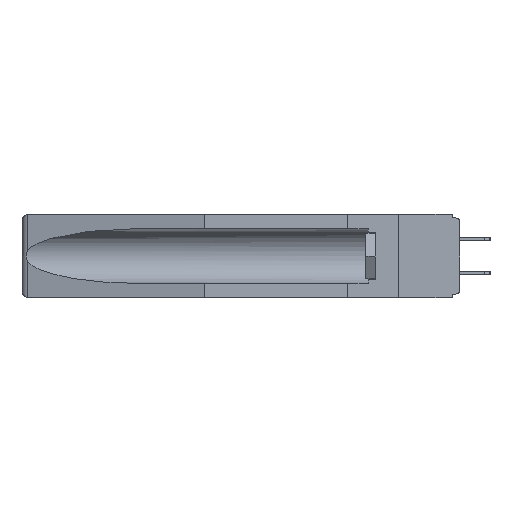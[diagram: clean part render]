
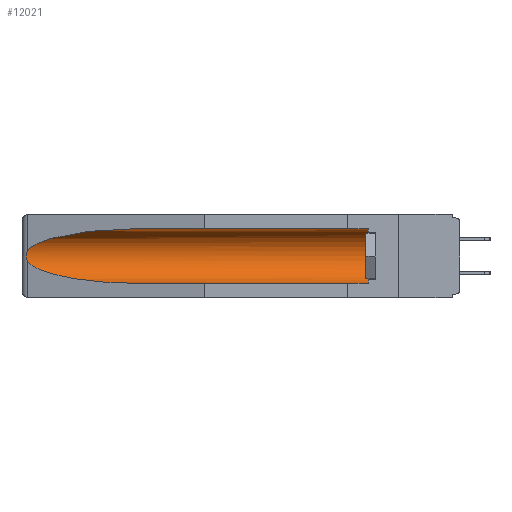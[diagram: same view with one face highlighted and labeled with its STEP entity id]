
A CAD part, left-side view. The second image highlights one B-rep face of the part: STEP entity #12021.
In plain terms, the highlighted cylindrical face has radius 2.857 mm (diameter 5.715 mm), a partial arc.
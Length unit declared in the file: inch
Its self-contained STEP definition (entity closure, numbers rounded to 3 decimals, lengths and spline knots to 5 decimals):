
#26 = EDGE_CURVE ( 'NONE', #24236, #4493, #21362, .T. ) ;
#445 = CARTESIAN_POINT ( 'NONE',  ( 0.155, 1.07973, -0.284 ) ) ;
#746 = DIRECTION ( 'NONE',  ( 0., -1., 0. ) ) ;
#1414 = AXIS2_PLACEMENT_3D ( 'NONE', #9236, #23745, #15819 ) ;
#2768 = CARTESIAN_POINT ( 'NONE',  ( 0.26597, 1.52961, -0.15275 ) ) ;
#2836 = CARTESIAN_POINT ( 'NONE',  ( 0.155, 1.07973, -0.059 ) ) ;
#3999 = DIRECTION ( 'NONE',  ( 0., 1., 0. ) ) ;
#4385 = CARTESIAN_POINT ( 'NONE',  ( 0.21114, 1.30732, -0.284 ) ) ;
#4493 = VERTEX_POINT ( 'NONE', #20191 ) ;
#4826 = CARTESIAN_POINT ( 'NONE',  ( 0.26537, 1.52718, -0.19328 ) ) ;
#4852 = CARTESIAN_POINT ( 'NONE',  ( 0.26537, 1.52718, -0.14972 ) ) ;
#5412 =( BOUNDED_CURVE ( )  B_SPLINE_CURVE ( 3, ( #15020, #23049, #4385, #445 ),
 .UNSPECIFIED., .F., .F. ) 
 B_SPLINE_CURVE_WITH_KNOTS ( ( 4, 4 ),
 ( 0.1948, 1.5708 ),
 .UNSPECIFIED. ) 
 CURVE ( )  GEOMETRIC_REPRESENTATION_ITEM ( )  RATIONAL_B_SPLINE_CURVE ( ( 1., 0.848, 0.848, 1. ) ) 
 REPRESENTATION_ITEM ( '' )  );
#5918 = CARTESIAN_POINT ( 'NONE',  ( 0.26537, 1.52718, -0.14972 ) ) ;
#6264 = ORIENTED_EDGE ( 'NONE', *, *, #21373, .T. ) ;
#7040 = VERTEX_POINT ( 'NONE', #2836 ) ;
#7216 = CARTESIAN_POINT ( 'NONE',  ( 0.155, 0.126, -0.284 ) ) ;
#7386 = ORIENTED_EDGE ( 'NONE', *, *, #23811, .F. ) ;
#8294 = VECTOR ( 'NONE', #3999, 39.37008 ) ;
#8612 = CARTESIAN_POINT ( 'NONE',  ( 0.26597, 1.5296, -0.19026 ) ) ;
#9236 = CARTESIAN_POINT ( 'NONE',  ( 0.155, -0.30754, -0.1715 ) ) ;
#9260 = CARTESIAN_POINT ( 'NONE',  ( 0.25451, 1.48313, -0.09465 ) ) ;
#9702 = ORIENTED_EDGE ( 'NONE', *, *, #26132, .T. ) ;
#9833 = CARTESIAN_POINT ( 'NONE',  ( 0.155, -0.30754, -0.284 ) ) ;
#11042 = CARTESIAN_POINT ( 'NONE',  ( 0.2673, 1.5327, -0.16383 ) ) ;
#11605 = CARTESIAN_POINT ( 'NONE',  ( 0.155, 1.07973, -0.284 ) ) ;
#11678 = FACE_OUTER_BOUND ( 'NONE', #24581, .T. ) ;
#12021 = ADVANCED_FACE ( 'NONE', ( #11678 ), #19457, .F. ) ;
#12266 = CARTESIAN_POINT ( 'NONE',  ( 0.21114, 1.30732, -0.059 ) ) ;
#12990 = CARTESIAN_POINT ( 'NONE',  ( 0.26537, 1.52718, -0.14972 ) ) ;
#14218 = LINE ( 'NONE', #22718, #14522 ) ;
#14522 = VECTOR ( 'NONE', #22549, 39.37008 ) ;
#14694 = VERTEX_POINT ( 'NONE', #11605 ) ;
#14932 = CARTESIAN_POINT ( 'NONE',  ( 0.2675, 1.53308, -0.16763 ) ) ;
#15020 = CARTESIAN_POINT ( 'NONE',  ( 0.26537, 1.52718, -0.19328 ) ) ;
#15023 = CARTESIAN_POINT ( 'NONE',  ( 0.26655, 1.53094, -0.18657 ) ) ;
#15447 = EDGE_CURVE ( 'NONE', #4493, #7040, #14218, .T. ) ;
#15819 = DIRECTION ( 'NONE',  ( 0., 0., 1. ) ) ;
#16822 = CARTESIAN_POINT ( 'NONE',  ( 0.2675, 1.53308, -0.17534 ) ) ;
#17211 = CARTESIAN_POINT ( 'NONE',  ( 0.155, 0.126, -0.1715 ) ) ;
#17786 = B_SPLINE_CURVE_WITH_KNOTS ( 'NONE', 3,
 ( #12990, #2768, #21065, #11042, #14932, #16822, #21321, #15023, #8612, #4826 ),
 .UNSPECIFIED., .F., .F.,
 ( 4, 2, 2, 2, 4 ),
 ( 0., 0.00029, 0.00058, 0.00087, 0.00117 ),
 .UNSPECIFIED. ) ;
#19131 = ORIENTED_EDGE ( 'NONE', *, *, #26, .T. ) ;
#19457 = CYLINDRICAL_SURFACE ( 'NONE', #1414, 0.1125 ) ;
#20191 = CARTESIAN_POINT ( 'NONE',  ( 0.155, 0.126, -0.059 ) ) ;
#20291 = VERTEX_POINT ( 'NONE', #26032 ) ;
#21065 = CARTESIAN_POINT ( 'NONE',  ( 0.26654, 1.53092, -0.15636 ) ) ;
#21321 = CARTESIAN_POINT ( 'NONE',  ( 0.2673, 1.53269, -0.17917 ) ) ;
#21362 = CIRCLE ( 'NONE', #22480, 0.1125 ) ;
#21373 = EDGE_CURVE ( 'NONE', #7040, #26527, #23735, .T. ) ;
#22405 = ORIENTED_EDGE ( 'NONE', *, *, #23442, .T. ) ;
#22480 = AXIS2_PLACEMENT_3D ( 'NONE', #17211, #746, #25216 ) ;
#22549 = DIRECTION ( 'NONE',  ( 0., 1., 0. ) ) ;
#22587 = CARTESIAN_POINT ( 'NONE',  ( 0.155, 1.07973, -0.059 ) ) ;
#22718 = CARTESIAN_POINT ( 'NONE',  ( 0.155, -0.30754, -0.059 ) ) ;
#23049 = CARTESIAN_POINT ( 'NONE',  ( 0.25451, 1.48313, -0.24835 ) ) ;
#23442 = EDGE_CURVE ( 'NONE', #20291, #14694, #5412, .T. ) ;
#23735 =( BOUNDED_CURVE ( )  B_SPLINE_CURVE ( 3, ( #22587, #12266, #9260, #4852 ),
 .UNSPECIFIED., .F., .F. ) 
 B_SPLINE_CURVE_WITH_KNOTS ( ( 4, 4 ),
 ( 4.71239, 6.08839 ),
 .UNSPECIFIED. ) 
 CURVE ( )  GEOMETRIC_REPRESENTATION_ITEM ( )  RATIONAL_B_SPLINE_CURVE ( ( 1., 0.848, 0.848, 1. ) ) 
 REPRESENTATION_ITEM ( '' )  );
#23745 = DIRECTION ( 'NONE',  ( 0., 1., 0. ) ) ;
#23811 = EDGE_CURVE ( 'NONE', #24236, #14694, #24078, .T. ) ;
#24078 = LINE ( 'NONE', #9833, #8294 ) ;
#24124 = ORIENTED_EDGE ( 'NONE', *, *, #15447, .T. ) ;
#24236 = VERTEX_POINT ( 'NONE', #7216 ) ;
#24581 = EDGE_LOOP ( 'NONE', ( #6264, #9702, #22405, #7386, #19131, #24124 ) ) ;
#25216 = DIRECTION ( 'NONE',  ( 0., 0., 1. ) ) ;
#26032 = CARTESIAN_POINT ( 'NONE',  ( 0.26537, 1.52718, -0.19328 ) ) ;
#26132 = EDGE_CURVE ( 'NONE', #26527, #20291, #17786, .T. ) ;
#26527 = VERTEX_POINT ( 'NONE', #5918 ) ;
